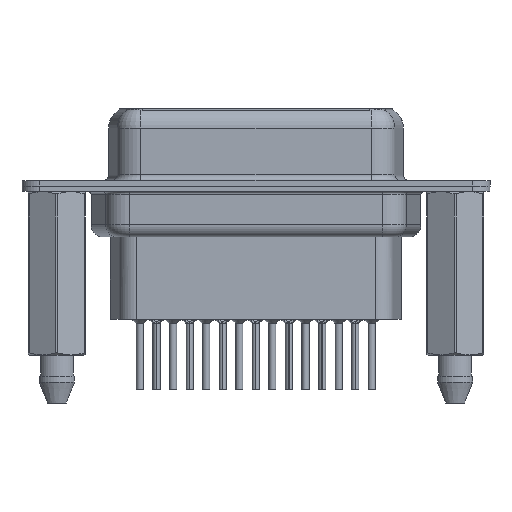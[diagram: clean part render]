
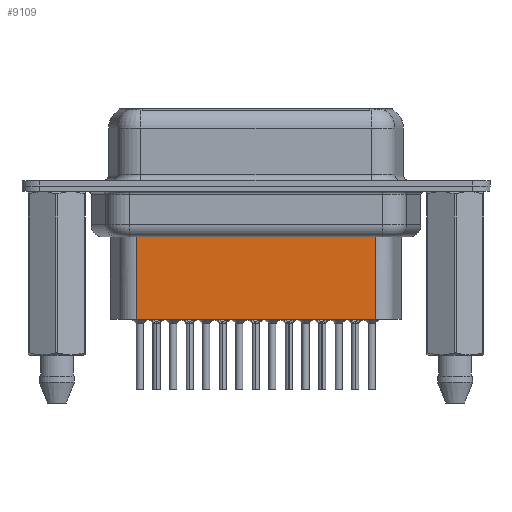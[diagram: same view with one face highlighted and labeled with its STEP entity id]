
A CAD part, front view. The second image highlights one B-rep face of the part: STEP entity #9109.
In plain terms, the highlighted planar face has unit normal (0, -1, 0).
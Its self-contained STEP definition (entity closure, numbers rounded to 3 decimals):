
#1439 = VERTEX_POINT ( 'NONE', #19572 ) ;
#1633 = CARTESIAN_POINT ( 'NONE',  ( 6.681, -3.5, -11.15 ) ) ;
#1756 = CARTESIAN_POINT ( 'NONE',  ( 6.434, -3.5, -4.097 ) ) ;
#1942 = EDGE_LOOP ( 'NONE', ( #22801, #3556, #24089, #11019 ) ) ;
#2008 = PLANE ( 'NONE',  #19741 ) ;
#3541 = LINE ( 'NONE', #1633, #24459 ) ;
#3556 = ORIENTED_EDGE ( 'NONE', *, *, #17326, .T. ) ;
#4035 = DIRECTION ( 'NONE',  ( -1., 0., 0. ) ) ;
#5550 = EDGE_CURVE ( 'NONE', #10291, #17401, #19326, .T. ) ;
#5919 = EDGE_CURVE ( 'NONE', #17401, #1439, #3541, .T. ) ;
#7140 = DIRECTION ( 'NONE',  ( 0., 0., -1. ) ) ;
#7440 = VECTOR ( 'NONE', #24654, 1000. ) ;
#7643 = DIRECTION ( 'NONE',  ( 1., 0., 0. ) ) ;
#8253 = VECTOR ( 'NONE', #7140, 1000. ) ;
#9109 = ADVANCED_FACE ( 'NONE', ( #12877 ), #2008, .T. ) ;
#10291 = VERTEX_POINT ( 'NONE', #23493 ) ;
#11019 = ORIENTED_EDGE ( 'NONE', *, *, #5919, .F. ) ;
#11790 = CARTESIAN_POINT ( 'NONE',  ( 26.619, -3.5, -11.15 ) ) ;
#12877 = FACE_OUTER_BOUND ( 'NONE', #1942, .T. ) ;
#13584 = LINE ( 'NONE', #1756, #20760 ) ;
#15379 = CARTESIAN_POINT ( 'NONE',  ( 6.681, -3.5, -3.1 ) ) ;
#16910 = LINE ( 'NONE', #22603, #8253 ) ;
#17272 = DIRECTION ( 'NONE',  ( 0., -1., 0. ) ) ;
#17326 = EDGE_CURVE ( 'NONE', #10291, #17679, #13584, .T. ) ;
#17401 = VERTEX_POINT ( 'NONE', #11790 ) ;
#17679 = VERTEX_POINT ( 'NONE', #22435 ) ;
#18448 = EDGE_CURVE ( 'NONE', #17679, #1439, #16910, .T. ) ;
#19204 = CARTESIAN_POINT ( 'NONE',  ( 26.619, -3.5, -3.1 ) ) ;
#19326 = LINE ( 'NONE', #19204, #7440 ) ;
#19572 = CARTESIAN_POINT ( 'NONE',  ( 6.681, -3.5, -11.15 ) ) ;
#19741 = AXIS2_PLACEMENT_3D ( 'NONE', #15379, #17272, #7643 ) ;
#20760 = VECTOR ( 'NONE', #4035, 1000. ) ;
#22435 = CARTESIAN_POINT ( 'NONE',  ( 6.681, -3.5, -4.097 ) ) ;
#22603 = CARTESIAN_POINT ( 'NONE',  ( 6.681, -3.5, -3.1 ) ) ;
#22801 = ORIENTED_EDGE ( 'NONE', *, *, #5550, .F. ) ;
#22831 = DIRECTION ( 'NONE',  ( -1., 0., 0. ) ) ;
#23493 = CARTESIAN_POINT ( 'NONE',  ( 26.619, -3.5, -4.097 ) ) ;
#24089 = ORIENTED_EDGE ( 'NONE', *, *, #18448, .T. ) ;
#24459 = VECTOR ( 'NONE', #22831, 1000. ) ;
#24654 = DIRECTION ( 'NONE',  ( 0., 0., -1. ) ) ;
